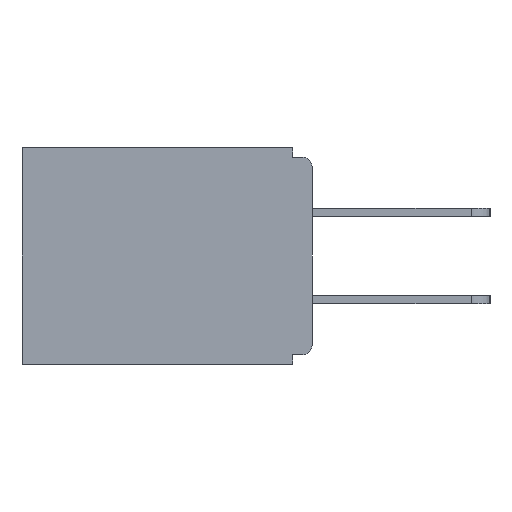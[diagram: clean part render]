
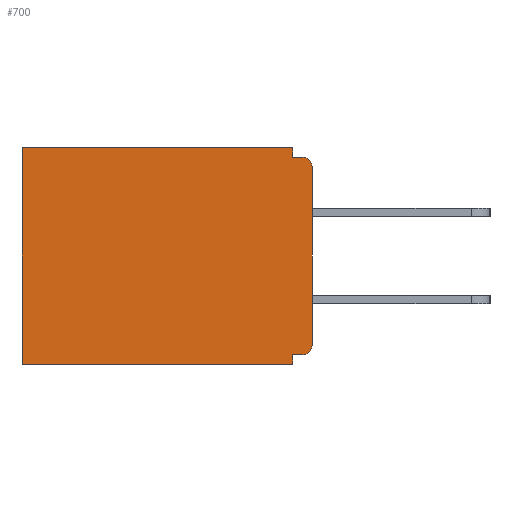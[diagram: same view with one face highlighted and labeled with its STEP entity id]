
A CAD part, left-side view. The second image highlights one B-rep face of the part: STEP entity #700.
In plain terms, the highlighted planar face has unit normal (-1, 0, 0).
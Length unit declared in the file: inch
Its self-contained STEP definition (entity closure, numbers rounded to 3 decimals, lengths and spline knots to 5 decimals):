
#164 = CARTESIAN_POINT ( 'NONE',  ( 0.298, 0.031, -0.343 ) ) ;
#604 = VECTOR ( 'NONE', #1448, 39.37008 ) ;
#700 = ADVANCED_FACE ( 'NONE', ( #4414 ), #9130, .F. ) ;
#873 = ORIENTED_EDGE ( 'NONE', *, *, #2405, .F. ) ;
#1034 = ORIENTED_EDGE ( 'NONE', *, *, #11199, .T. ) ;
#1274 = CIRCLE ( 'NONE', #8817, 0.015 ) ;
#1285 = AXIS2_PLACEMENT_3D ( 'NONE', #6137, #3809, #8313 ) ;
#1420 = EDGE_CURVE ( 'NONE', #2390, #6138, #10703, .T. ) ;
#1448 = DIRECTION ( 'NONE',  ( 0., 0., -1. ) ) ;
#1472 = CARTESIAN_POINT ( 'NONE',  ( 0.298, 0., 0. ) ) ;
#1852 = VERTEX_POINT ( 'NONE', #5180 ) ;
#1923 = VECTOR ( 'NONE', #2034, 39.37008 ) ;
#2034 = DIRECTION ( 'NONE',  ( 0., 1., 0. ) ) ;
#2156 = DIRECTION ( 'NONE',  ( -1., 0., 0. ) ) ;
#2390 = VERTEX_POINT ( 'NONE', #10927 ) ;
#2405 = EDGE_CURVE ( 'NONE', #6221, #7187, #4449, .T. ) ;
#2423 = EDGE_CURVE ( 'NONE', #1852, #8699, #1274, .T. ) ;
#2494 = DIRECTION ( 'NONE',  ( 0., 0., -1. ) ) ;
#2571 = VERTEX_POINT ( 'NONE', #7973 ) ;
#2586 = CARTESIAN_POINT ( 'NONE',  ( 0.298, 0.031, -0.328 ) ) ;
#2836 = CARTESIAN_POINT ( 'NONE',  ( 0.298, 0., -0.015 ) ) ;
#2875 = EDGE_CURVE ( 'NONE', #7187, #2571, #7390, .T. ) ;
#2887 = ORIENTED_EDGE ( 'NONE', *, *, #3145, .F. ) ;
#3145 = EDGE_CURVE ( 'NONE', #1852, #5230, #7939, .T. ) ;
#3502 = ORIENTED_EDGE ( 'NONE', *, *, #2875, .F. ) ;
#3809 = DIRECTION ( 'NONE',  ( -1., 0., 0. ) ) ;
#3855 = CARTESIAN_POINT ( 'NONE',  ( 0.298, 0.031, -0.343 ) ) ;
#3917 = DIRECTION ( 'NONE',  ( 1., 0., 0. ) ) ;
#3918 = DIRECTION ( 'NONE',  ( 0., 0., -1. ) ) ;
#3971 = DIRECTION ( 'NONE',  ( 0., -1., 0. ) ) ;
#4147 = VECTOR ( 'NONE', #3918, 39.37008 ) ;
#4385 = ORIENTED_EDGE ( 'NONE', *, *, #9788, .F. ) ;
#4395 = AXIS2_PLACEMENT_3D ( 'NONE', #1472, #3917, #11747 ) ;
#4414 = FACE_OUTER_BOUND ( 'NONE', #7978, .T. ) ;
#4449 = LINE ( 'NONE', #13203, #10054 ) ;
#4717 = DIRECTION ( 'NONE',  ( 0., 0., -1. ) ) ;
#4765 = VECTOR ( 'NONE', #2494, 39.37008 ) ;
#4801 = VECTOR ( 'NONE', #3971, 39.37008 ) ;
#5083 = CIRCLE ( 'NONE', #1285, 0.015 ) ;
#5180 = CARTESIAN_POINT ( 'NONE',  ( 0.298, 0., -0.03 ) ) ;
#5230 = VERTEX_POINT ( 'NONE', #5705 ) ;
#5705 = CARTESIAN_POINT ( 'NONE',  ( 0.298, 0., -0.313 ) ) ;
#6137 = CARTESIAN_POINT ( 'NONE',  ( 0.298, 0.015, -0.313 ) ) ;
#6138 = VERTEX_POINT ( 'NONE', #8281 ) ;
#6166 = VECTOR ( 'NONE', #4717, 39.37008 ) ;
#6221 = VERTEX_POINT ( 'NONE', #6733 ) ;
#6417 = CARTESIAN_POINT ( 'NONE',  ( 0.298, 0., 0. ) ) ;
#6676 = LINE ( 'NONE', #164, #4765 ) ;
#6733 = CARTESIAN_POINT ( 'NONE',  ( 0.298, 0.015, -0.328 ) ) ;
#6827 = EDGE_CURVE ( 'NONE', #6138, #11362, #7265, .T. ) ;
#7000 = CARTESIAN_POINT ( 'NONE',  ( 0.298, 0., -0.343 ) ) ;
#7156 = CARTESIAN_POINT ( 'NONE',  ( 0.298, 0.031, -0.015 ) ) ;
#7187 = VERTEX_POINT ( 'NONE', #2586 ) ;
#7265 = LINE ( 'NONE', #13863, #4147 ) ;
#7390 = LINE ( 'NONE', #3855, #604 ) ;
#7673 = CARTESIAN_POINT ( 'NONE',  ( 0.298, 0.015, -0.015 ) ) ;
#7839 = EDGE_CURVE ( 'NONE', #12493, #8699, #8496, .T. ) ;
#7939 = LINE ( 'NONE', #10653, #6166 ) ;
#7944 = ORIENTED_EDGE ( 'NONE', *, *, #6827, .T. ) ;
#7973 = CARTESIAN_POINT ( 'NONE',  ( 0.298, 0.031, -0.343 ) ) ;
#7978 = EDGE_LOOP ( 'NONE', ( #14104, #11597, #4385, #14391, #7944, #9837, #3502, #873, #1034, #2887 ) ) ;
#8066 = LINE ( 'NONE', #7000, #8226 ) ;
#8226 = VECTOR ( 'NONE', #12634, 39.37008 ) ;
#8281 = CARTESIAN_POINT ( 'NONE',  ( 0.298, 0.46, 0. ) ) ;
#8313 = DIRECTION ( 'NONE',  ( 0., 0., -1. ) ) ;
#8496 = LINE ( 'NONE', #2836, #4801 ) ;
#8699 = VERTEX_POINT ( 'NONE', #7673 ) ;
#8817 = AXIS2_PLACEMENT_3D ( 'NONE', #9911, #2156, #9853 ) ;
#9130 = PLANE ( 'NONE',  #4395 ) ;
#9788 = EDGE_CURVE ( 'NONE', #2390, #12493, #6676, .T. ) ;
#9837 = ORIENTED_EDGE ( 'NONE', *, *, #11630, .F. ) ;
#9853 = DIRECTION ( 'NONE',  ( 0., 0., -1. ) ) ;
#9911 = CARTESIAN_POINT ( 'NONE',  ( 0.298, 0.015, -0.03 ) ) ;
#10054 = VECTOR ( 'NONE', #13143, 39.37008 ) ;
#10653 = CARTESIAN_POINT ( 'NONE',  ( 0.298, 0., 0. ) ) ;
#10703 = LINE ( 'NONE', #6417, #1923 ) ;
#10927 = CARTESIAN_POINT ( 'NONE',  ( 0.298, 0.031, 0. ) ) ;
#11199 = EDGE_CURVE ( 'NONE', #6221, #5230, #5083, .T. ) ;
#11362 = VERTEX_POINT ( 'NONE', #11639 ) ;
#11597 = ORIENTED_EDGE ( 'NONE', *, *, #7839, .F. ) ;
#11630 = EDGE_CURVE ( 'NONE', #2571, #11362, #8066, .T. ) ;
#11639 = CARTESIAN_POINT ( 'NONE',  ( 0.298, 0.46, -0.343 ) ) ;
#11747 = DIRECTION ( 'NONE',  ( 0., 0., -1. ) ) ;
#12493 = VERTEX_POINT ( 'NONE', #7156 ) ;
#12634 = DIRECTION ( 'NONE',  ( 0., 1., 0. ) ) ;
#13143 = DIRECTION ( 'NONE',  ( 0., 1., 0. ) ) ;
#13203 = CARTESIAN_POINT ( 'NONE',  ( 0.298, 0., -0.328 ) ) ;
#13863 = CARTESIAN_POINT ( 'NONE',  ( 0.298, 0.46, 0. ) ) ;
#14104 = ORIENTED_EDGE ( 'NONE', *, *, #2423, .T. ) ;
#14391 = ORIENTED_EDGE ( 'NONE', *, *, #1420, .T. ) ;
